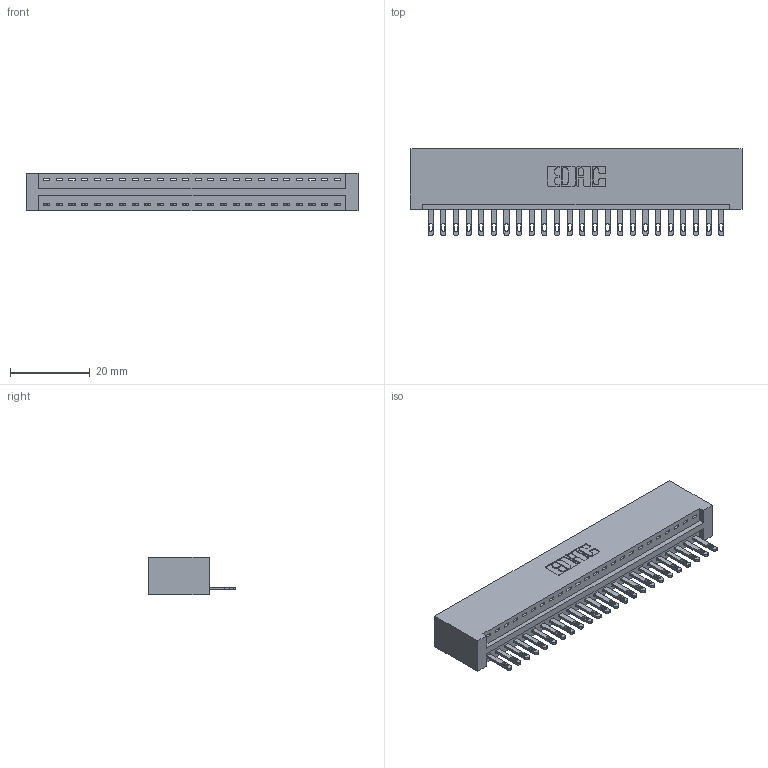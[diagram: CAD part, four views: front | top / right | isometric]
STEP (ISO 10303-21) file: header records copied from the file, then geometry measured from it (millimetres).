
FILE_DESCRIPTION (( 'STEP AP203' ), '1' );
FILE_NAME ('346-024-500-101.STEP', '2018-08-21T02:32:01', ( '' ), ( '' ), 'SwSTEP 2.0', 'SolidWorks 2016', '' );
FILE_SCHEMA (( 'CONFIG_CONTROL_DESIGN' ));
Length unit declared in the file: inch
Products named in the file (3): 346 Part_No Mounting Lugs; 345-292-001_345-293-100; 346-024-500-101
Assembly tree (25 placements, depth 2):
  346-024-500-101
    346 Part_No Mounting Lugs
    345-292-001_345-293-100  x24
Bounding box: 83.44 x 21.84 x 9.4 mm (x, y, z)
Volume: 8427.2 mm3; surface area: 10469.7 mm2
Topology: 25 solids, 25 shells, 1410 faces, 4337 edges, 2890 vertices
Faces by surface type: plane 888, cylinder 522
Entity records: 16971 total; most frequent: CARTESIAN_POINT 2920, ORIENTED_EDGE 2878, DIRECTION 2595, EDGE_CURVE 1439, LINE 1215, VECTOR 1215, VERTEX_POINT 958, AXIS2_PLACEMENT_3D 690
